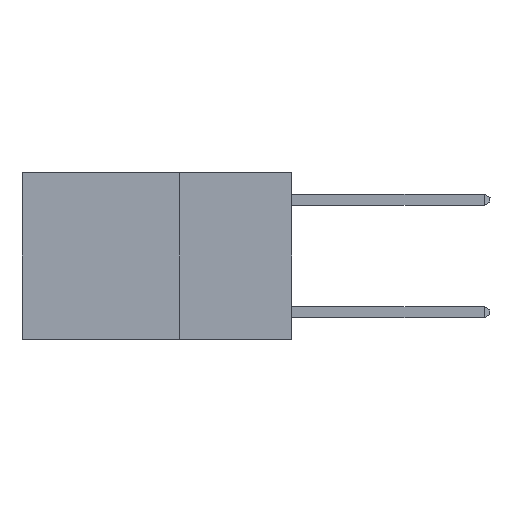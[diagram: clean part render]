
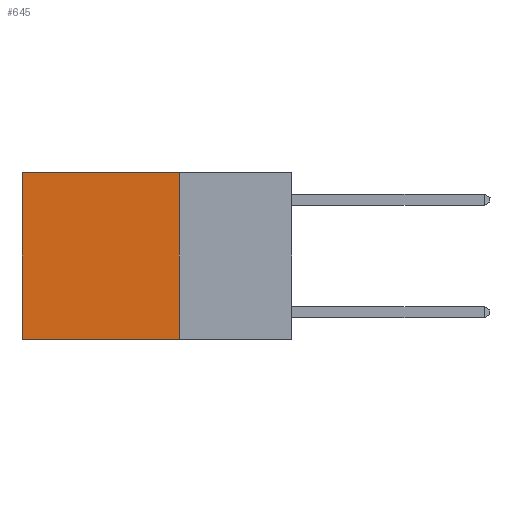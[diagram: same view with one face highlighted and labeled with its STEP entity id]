
A CAD part, left-side view. The second image highlights one B-rep face of the part: STEP entity #645.
In plain terms, the highlighted planar face has unit normal (-1, 0, 0).
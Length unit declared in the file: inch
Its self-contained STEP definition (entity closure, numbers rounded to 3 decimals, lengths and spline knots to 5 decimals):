
#478 = CARTESIAN_POINT ( 'NONE',  ( 0.2625, 0.25, -0.37 ) ) ;
#504 = ORIENTED_EDGE ( 'NONE', *, *, #14003, .T. ) ;
#567 = ORIENTED_EDGE ( 'NONE', *, *, #4995, .F. ) ;
#645 = ADVANCED_FACE ( 'NONE', ( #8523 ), #9880, .F. ) ;
#688 = ORIENTED_EDGE ( 'NONE', *, *, #14095, .T. ) ;
#751 = CARTESIAN_POINT ( 'NONE',  ( 0.2625, 0.25, -0.37 ) ) ;
#1703 = VERTEX_POINT ( 'NONE', #5005 ) ;
#1783 = AXIS2_PLACEMENT_3D ( 'NONE', #9822, #3863, #9863 ) ;
#3460 = ORIENTED_EDGE ( 'NONE', *, *, #4066, .F. ) ;
#3863 = DIRECTION ( 'NONE',  ( 1., 0., 0. ) ) ;
#3944 = DIRECTION ( 'NONE',  ( 0., 1., 0. ) ) ;
#4066 = EDGE_CURVE ( 'NONE', #9281, #1703, #5650, .T. ) ;
#4071 = CARTESIAN_POINT ( 'NONE',  ( 0.2625, 0.25, 0. ) ) ;
#4187 = LINE ( 'NONE', #10543, #13189 ) ;
#4434 = DIRECTION ( 'NONE',  ( 0., 0., -1. ) ) ;
#4619 = CARTESIAN_POINT ( 'NONE',  ( 0.2625, 0.6, 0. ) ) ;
#4995 = EDGE_CURVE ( 'NONE', #10732, #9281, #10259, .T. ) ;
#5005 = CARTESIAN_POINT ( 'NONE',  ( 0.2625, 0.6, -0.37 ) ) ;
#5650 = LINE ( 'NONE', #751, #8243 ) ;
#6307 = LINE ( 'NONE', #4619, #12025 ) ;
#6492 = EDGE_LOOP ( 'NONE', ( #504, #3460, #567, #688 ) ) ;
#7658 = DIRECTION ( 'NONE',  ( 0., 1., 0. ) ) ;
#8030 = CARTESIAN_POINT ( 'NONE',  ( 0.2625, 0.6, 0. ) ) ;
#8243 = VECTOR ( 'NONE', #7658, 39.37008 ) ;
#8523 = FACE_OUTER_BOUND ( 'NONE', #6492, .T. ) ;
#9281 = VERTEX_POINT ( 'NONE', #478 ) ;
#9822 = CARTESIAN_POINT ( 'NONE',  ( 0.2625, 0.25, 0. ) ) ;
#9863 = DIRECTION ( 'NONE',  ( 0., 0., -1. ) ) ;
#9880 = PLANE ( 'NONE',  #1783 ) ;
#9907 = VECTOR ( 'NONE', #4434, 39.37008 ) ;
#9930 = CARTESIAN_POINT ( 'NONE',  ( 0.2625, 0.25, 0. ) ) ;
#10259 = LINE ( 'NONE', #9930, #9907 ) ;
#10543 = CARTESIAN_POINT ( 'NONE',  ( 0.2625, 0.25, 0. ) ) ;
#10732 = VERTEX_POINT ( 'NONE', #4071 ) ;
#11184 = DIRECTION ( 'NONE',  ( 0., 0., -1. ) ) ;
#12025 = VECTOR ( 'NONE', #11184, 39.37008 ) ;
#12054 = VERTEX_POINT ( 'NONE', #8030 ) ;
#13189 = VECTOR ( 'NONE', #3944, 39.37008 ) ;
#14003 = EDGE_CURVE ( 'NONE', #12054, #1703, #6307, .T. ) ;
#14095 = EDGE_CURVE ( 'NONE', #10732, #12054, #4187, .T. ) ;
